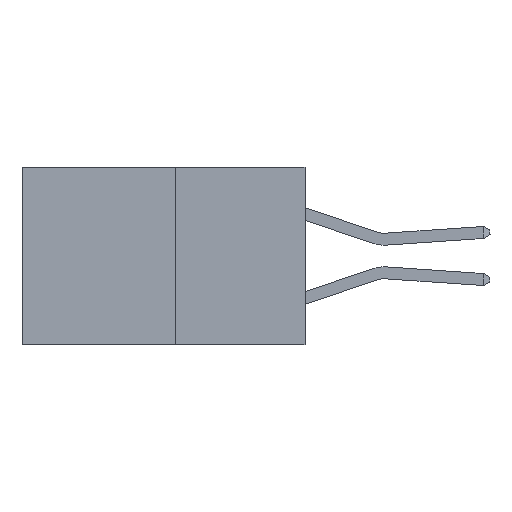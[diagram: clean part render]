
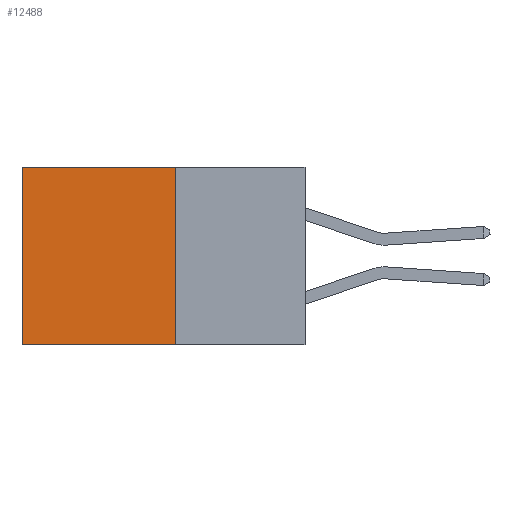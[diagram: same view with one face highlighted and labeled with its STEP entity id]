
A CAD part, left-side view. The second image highlights one B-rep face of the part: STEP entity #12488.
In plain terms, the highlighted planar face has unit normal (-1, 0, 0).
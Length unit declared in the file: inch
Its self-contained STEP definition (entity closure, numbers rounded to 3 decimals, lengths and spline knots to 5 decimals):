
#1183 = CARTESIAN_POINT ( 'NONE',  ( 0.277, 0.27, 0. ) ) ;
#2530 = LINE ( 'NONE', #1183, #13333 ) ;
#3388 = FACE_OUTER_BOUND ( 'NONE', #16757, .T. ) ;
#4286 = VECTOR ( 'NONE', #17143, 39.37008 ) ;
#4566 = CARTESIAN_POINT ( 'NONE',  ( 0.277, 0.27, -0.37 ) ) ;
#4787 = VECTOR ( 'NONE', #13954, 39.37008 ) ;
#5248 = CARTESIAN_POINT ( 'NONE',  ( 0.277, 0.59, -0.37 ) ) ;
#5802 = CARTESIAN_POINT ( 'NONE',  ( 0.277, 0.27, -0.37 ) ) ;
#5938 = DIRECTION ( 'NONE',  ( 1., 0., 0. ) ) ;
#6179 = ORIENTED_EDGE ( 'NONE', *, *, #13015, .T. ) ;
#6727 = CARTESIAN_POINT ( 'NONE',  ( 0.277, 0.27, 0. ) ) ;
#6971 = CARTESIAN_POINT ( 'NONE',  ( 0.277, 0.27, -0.37 ) ) ;
#8000 = LINE ( 'NONE', #5802, #4787 ) ;
#8102 = ORIENTED_EDGE ( 'NONE', *, *, #10877, .T. ) ;
#8611 = LINE ( 'NONE', #5248, #15753 ) ;
#8631 = VERTEX_POINT ( 'NONE', #6971 ) ;
#8769 = LINE ( 'NONE', #13206, #4286 ) ;
#8774 = VERTEX_POINT ( 'NONE', #6727 ) ;
#9317 = DIRECTION ( 'NONE',  ( 0., 0., -1. ) ) ;
#10877 = EDGE_CURVE ( 'NONE', #16447, #13698, #8611, .T. ) ;
#11545 = AXIS2_PLACEMENT_3D ( 'NONE', #4566, #5938, #15412 ) ;
#12053 = EDGE_CURVE ( 'NONE', #8774, #8631, #8769, .T. ) ;
#12488 = ADVANCED_FACE ( 'NONE', ( #3388 ), #12676, .F. ) ;
#12676 = PLANE ( 'NONE',  #11545 ) ;
#13015 = EDGE_CURVE ( 'NONE', #8774, #16447, #2530, .T. ) ;
#13206 = CARTESIAN_POINT ( 'NONE',  ( 0.277, 0.27, -0.37 ) ) ;
#13333 = VECTOR ( 'NONE', #14755, 39.37008 ) ;
#13427 = CARTESIAN_POINT ( 'NONE',  ( 0.277, 0.59, -0.37 ) ) ;
#13698 = VERTEX_POINT ( 'NONE', #13427 ) ;
#13954 = DIRECTION ( 'NONE',  ( 0., 1., 0. ) ) ;
#13989 = EDGE_CURVE ( 'NONE', #8631, #13698, #8000, .T. ) ;
#14755 = DIRECTION ( 'NONE',  ( 0., 1., 0. ) ) ;
#15412 = DIRECTION ( 'NONE',  ( 0., 0., -1. ) ) ;
#15678 = ORIENTED_EDGE ( 'NONE', *, *, #13989, .F. ) ;
#15753 = VECTOR ( 'NONE', #9317, 39.37008 ) ;
#16447 = VERTEX_POINT ( 'NONE', #17270 ) ;
#16492 = ORIENTED_EDGE ( 'NONE', *, *, #12053, .F. ) ;
#16757 = EDGE_LOOP ( 'NONE', ( #8102, #15678, #16492, #6179 ) ) ;
#17143 = DIRECTION ( 'NONE',  ( 0., 0., -1. ) ) ;
#17270 = CARTESIAN_POINT ( 'NONE',  ( 0.277, 0.59, 0. ) ) ;
